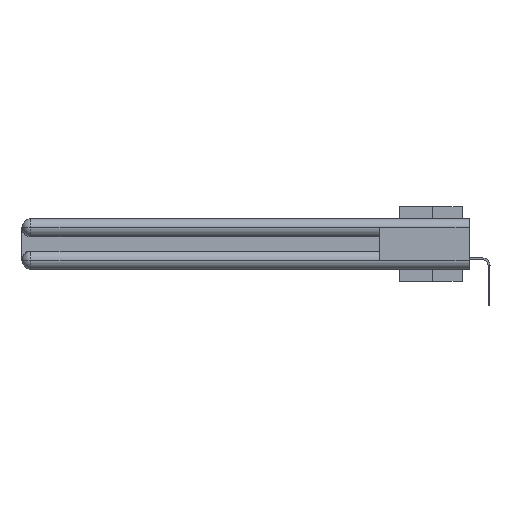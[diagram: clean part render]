
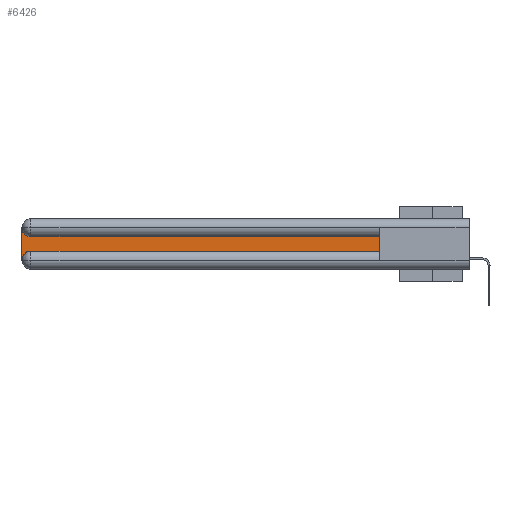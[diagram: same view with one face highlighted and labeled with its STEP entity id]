
A CAD part, left-side view. The second image highlights one B-rep face of the part: STEP entity #6426.
In plain terms, the highlighted planar face has unit normal (-1, 0, 0).
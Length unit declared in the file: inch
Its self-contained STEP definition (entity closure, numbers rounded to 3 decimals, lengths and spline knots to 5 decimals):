
#144 = DIRECTION ( 'NONE',  ( 1., 0., 0. ) ) ;
#1761 = CARTESIAN_POINT ( 'NONE',  ( 0.075, 3., -0.1225 ) ) ;
#1989 = VERTEX_POINT ( 'NONE', #13284 ) ;
#4163 = AXIS2_PLACEMENT_3D ( 'NONE', #1761, #29256, #20646 ) ;
#4620 = LINE ( 'NONE', #27138, #33594 ) ;
#4861 = EDGE_CURVE ( 'NONE', #15266, #18915, #4620, .T. ) ;
#5560 = ORIENTED_EDGE ( 'NONE', *, *, #13616, .T. ) ;
#5744 = CARTESIAN_POINT ( 'NONE',  ( 0.075, 2.94, -0.0625 ) ) ;
#5781 = DIRECTION ( 'NONE',  ( 0., 0., -1. ) ) ;
#6426 = ADVANCED_FACE ( 'NONE', ( #30830 ), #15486, .F. ) ;
#7436 = EDGE_CURVE ( 'NONE', #18915, #26883, #23829, .T. ) ;
#8253 = ORIENTED_EDGE ( 'NONE', *, *, #35037, .T. ) ;
#8718 = VERTEX_POINT ( 'NONE', #17959 ) ;
#8882 = CARTESIAN_POINT ( 'NONE',  ( 0.075, 0.6, -0.1225 ) ) ;
#9598 = CIRCLE ( 'NONE', #12891, 0.06 ) ;
#12891 = AXIS2_PLACEMENT_3D ( 'NONE', #16612, #144, #5781 ) ;
#13030 = LINE ( 'NONE', #15827, #32912 ) ;
#13284 = CARTESIAN_POINT ( 'NONE',  ( 0.075, 2.94, -0.1225 ) ) ;
#13616 = EDGE_CURVE ( 'NONE', #8718, #15266, #9598, .T. ) ;
#14213 = CARTESIAN_POINT ( 'NONE',  ( 0.075, 0.6, -0.2175 ) ) ;
#15266 = VERTEX_POINT ( 'NONE', #31152 ) ;
#15486 = PLANE ( 'NONE',  #4163 ) ;
#15827 = CARTESIAN_POINT ( 'NONE',  ( 0.075, 0.6, -0.1225 ) ) ;
#15859 = CARTESIAN_POINT ( 'NONE',  ( 0.075, 3., -0.0625 ) ) ;
#16612 = CARTESIAN_POINT ( 'NONE',  ( 0.075, 2.94, -0.2775 ) ) ;
#16759 = EDGE_CURVE ( 'NONE', #26883, #1989, #13030, .T. ) ;
#16806 = DIRECTION ( 'NONE',  ( 0., 0., -1. ) ) ;
#17382 = CARTESIAN_POINT ( 'NONE',  ( 0.075, 0.6, -0.2175 ) ) ;
#17959 = CARTESIAN_POINT ( 'NONE',  ( 0.075, 3., -0.2775 ) ) ;
#18275 = DIRECTION ( 'NONE',  ( 0., 0., -1. ) ) ;
#18915 = VERTEX_POINT ( 'NONE', #17382 ) ;
#20016 = LINE ( 'NONE', #20913, #27410 ) ;
#20646 = DIRECTION ( 'NONE',  ( 0., 0., -1. ) ) ;
#20913 = CARTESIAN_POINT ( 'NONE',  ( 0.075, 3., -0.2175 ) ) ;
#21518 = EDGE_CURVE ( 'NONE', #1989, #28278, #35828, .T. ) ;
#23829 = LINE ( 'NONE', #14213, #27293 ) ;
#24045 = ORIENTED_EDGE ( 'NONE', *, *, #7436, .T. ) ;
#24458 = ORIENTED_EDGE ( 'NONE', *, *, #4861, .T. ) ;
#24571 = AXIS2_PLACEMENT_3D ( 'NONE', #5744, #30594, #16806 ) ;
#26883 = VERTEX_POINT ( 'NONE', #8882 ) ;
#27138 = CARTESIAN_POINT ( 'NONE',  ( 0.075, 0.6, -0.2175 ) ) ;
#27293 = VECTOR ( 'NONE', #33074, 39.37008 ) ;
#27410 = VECTOR ( 'NONE', #18275, 39.37008 ) ;
#28278 = VERTEX_POINT ( 'NONE', #15859 ) ;
#29256 = DIRECTION ( 'NONE',  ( 1., 0., 0. ) ) ;
#29604 = DIRECTION ( 'NONE',  ( 0., 1., 0. ) ) ;
#30594 = DIRECTION ( 'NONE',  ( 1., 0., 0. ) ) ;
#30781 = EDGE_LOOP ( 'NONE', ( #32794, #32171, #8253, #5560, #24458, #24045 ) ) ;
#30830 = FACE_OUTER_BOUND ( 'NONE', #30781, .T. ) ;
#31152 = CARTESIAN_POINT ( 'NONE',  ( 0.075, 2.94, -0.2175 ) ) ;
#32171 = ORIENTED_EDGE ( 'NONE', *, *, #21518, .T. ) ;
#32794 = ORIENTED_EDGE ( 'NONE', *, *, #16759, .T. ) ;
#32912 = VECTOR ( 'NONE', #29604, 39.37008 ) ;
#33074 = DIRECTION ( 'NONE',  ( 0., 0., 1. ) ) ;
#33594 = VECTOR ( 'NONE', #35293, 39.37008 ) ;
#35037 = EDGE_CURVE ( 'NONE', #28278, #8718, #20016, .T. ) ;
#35293 = DIRECTION ( 'NONE',  ( 0., -1., 0. ) ) ;
#35828 = CIRCLE ( 'NONE', #24571, 0.06 ) ;
